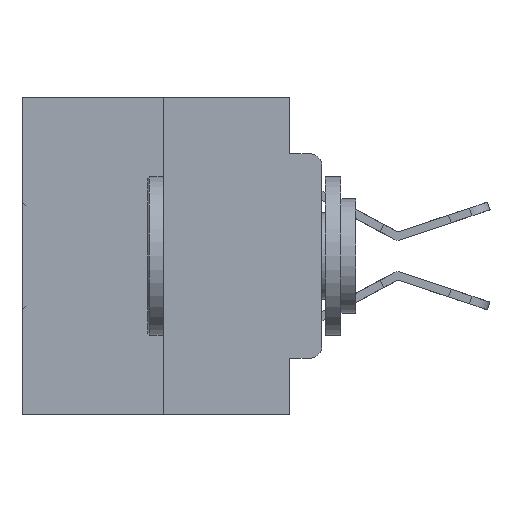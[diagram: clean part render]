
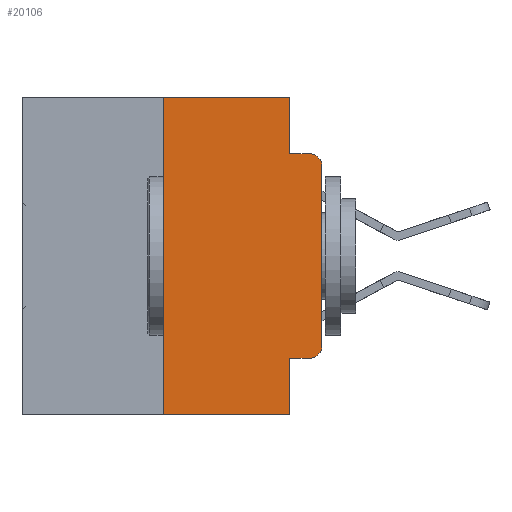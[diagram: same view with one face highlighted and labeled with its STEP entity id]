
A CAD part, left-side view. The second image highlights one B-rep face of the part: STEP entity #20106.
In plain terms, the highlighted planar face has unit normal (-1, 0, 0).
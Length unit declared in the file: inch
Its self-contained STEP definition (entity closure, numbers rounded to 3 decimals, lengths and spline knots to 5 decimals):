
#371 = LINE ( 'NONE', #14412, #5824 ) ;
#836 = LINE ( 'NONE', #15766, #27241 ) ;
#962 = AXIS2_PLACEMENT_3D ( 'NONE', #31679, #16989, #1334 ) ;
#1334 = DIRECTION ( 'NONE',  ( 0., 0., -1. ) ) ;
#1443 = CARTESIAN_POINT ( 'NONE',  ( 0., 0.25, 0. ) ) ;
#1531 = CIRCLE ( 'NONE', #962, 0.02 ) ;
#1955 = ORIENTED_EDGE ( 'NONE', *, *, #29568, .F. ) ;
#3043 = VECTOR ( 'NONE', #22817, 39.37008 ) ;
#3607 = LINE ( 'NONE', #12503, #16623 ) ;
#3695 = DIRECTION ( 'NONE',  ( 0., -1., 0. ) ) ;
#4086 = EDGE_CURVE ( 'NONE', #24337, #12798, #836, .T. ) ;
#4461 = ORIENTED_EDGE ( 'NONE', *, *, #20427, .T. ) ;
#5219 = PLANE ( 'NONE',  #29538 ) ;
#5430 = EDGE_CURVE ( 'NONE', #26293, #6382, #20924, .T. ) ;
#5565 = CARTESIAN_POINT ( 'NONE',  ( 0., 0.02, -0.1085 ) ) ;
#5824 = VECTOR ( 'NONE', #6723, 39.37008 ) ;
#6382 = VERTEX_POINT ( 'NONE', #22737 ) ;
#6723 = DIRECTION ( 'NONE',  ( 0., -1., 0. ) ) ;
#7226 = VECTOR ( 'NONE', #17178, 39.37008 ) ;
#7345 = CIRCLE ( 'NONE', #23878, 0.02 ) ;
#7368 = ORIENTED_EDGE ( 'NONE', *, *, #8764, .F. ) ;
#7575 = CARTESIAN_POINT ( 'NONE',  ( 0., 0.25, 0. ) ) ;
#8210 = DIRECTION ( 'NONE',  ( 0., 0., -1. ) ) ;
#8244 = CARTESIAN_POINT ( 'NONE',  ( 0., 0.051, 0. ) ) ;
#8764 = EDGE_CURVE ( 'NONE', #10915, #15025, #371, .T. ) ;
#9441 = VECTOR ( 'NONE', #12786, 39.37008 ) ;
#9856 = EDGE_CURVE ( 'NONE', #26293, #10915, #29400, .T. ) ;
#9999 = LINE ( 'NONE', #26650, #16008 ) ;
#10063 = LINE ( 'NONE', #20355, #3043 ) ;
#10625 = EDGE_CURVE ( 'NONE', #26866, #32102, #7345, .T. ) ;
#10708 = VERTEX_POINT ( 'NONE', #13634 ) ;
#10915 = VERTEX_POINT ( 'NONE', #1443 ) ;
#11816 = ORIENTED_EDGE ( 'NONE', *, *, #26730, .T. ) ;
#12371 = CARTESIAN_POINT ( 'NONE',  ( 0., 0.473, -0.5 ) ) ;
#12503 = CARTESIAN_POINT ( 'NONE',  ( 0., 0., 0. ) ) ;
#12786 = DIRECTION ( 'NONE',  ( 0., 0., 1. ) ) ;
#12798 = VERTEX_POINT ( 'NONE', #30124 ) ;
#13430 = CARTESIAN_POINT ( 'NONE',  ( 0., 0., -0.3915 ) ) ;
#13448 = ORIENTED_EDGE ( 'NONE', *, *, #17779, .F. ) ;
#13587 = LINE ( 'NONE', #8244, #19589 ) ;
#13634 = CARTESIAN_POINT ( 'NONE',  ( 0., 0.051, -0.0885 ) ) ;
#14412 = CARTESIAN_POINT ( 'NONE',  ( 0., 0.473, 0. ) ) ;
#15025 = VERTEX_POINT ( 'NONE', #18562 ) ;
#15657 = DIRECTION ( 'NONE',  ( 0., 0., -1. ) ) ;
#15766 = CARTESIAN_POINT ( 'NONE',  ( 0., 0.051, -0.4115 ) ) ;
#16008 = VECTOR ( 'NONE', #29107, 39.37008 ) ;
#16623 = VECTOR ( 'NONE', #17682, 39.37008 ) ;
#16989 = DIRECTION ( 'NONE',  ( -1., 0., 0. ) ) ;
#17178 = DIRECTION ( 'NONE',  ( 0., -1., 0. ) ) ;
#17479 = FACE_OUTER_BOUND ( 'NONE', #19697, .T. ) ;
#17682 = DIRECTION ( 'NONE',  ( 0., 0., 1. ) ) ;
#17779 = EDGE_CURVE ( 'NONE', #15025, #10708, #13587, .T. ) ;
#18487 = DIRECTION ( 'NONE',  ( 0., 0., -1. ) ) ;
#18562 = CARTESIAN_POINT ( 'NONE',  ( 0., 0.051, 0. ) ) ;
#19453 = ORIENTED_EDGE ( 'NONE', *, *, #28633, .F. ) ;
#19589 = VECTOR ( 'NONE', #18487, 39.37008 ) ;
#19697 = EDGE_LOOP ( 'NONE', ( #11816, #31633, #19453, #13448, #7368, #21046, #27466, #1955, #29000, #4461 ) ) ;
#20106 = ADVANCED_FACE ( 'NONE', ( #17479 ), #5219, .F. ) ;
#20355 = CARTESIAN_POINT ( 'NONE',  ( 0., 0.051, -0.0885 ) ) ;
#20427 = EDGE_CURVE ( 'NONE', #12798, #22622, #1531, .T. ) ;
#20924 = LINE ( 'NONE', #12371, #7226 ) ;
#20938 = CARTESIAN_POINT ( 'NONE',  ( 0., 0.25, -0.5 ) ) ;
#21046 = ORIENTED_EDGE ( 'NONE', *, *, #9856, .F. ) ;
#22622 = VERTEX_POINT ( 'NONE', #13430 ) ;
#22737 = CARTESIAN_POINT ( 'NONE',  ( 0., 0.051, -0.5 ) ) ;
#22817 = DIRECTION ( 'NONE',  ( 0., -1., 0. ) ) ;
#23448 = DIRECTION ( 'NONE',  ( -1., 0., 0. ) ) ;
#23878 = AXIS2_PLACEMENT_3D ( 'NONE', #5565, #23448, #8210 ) ;
#24337 = VERTEX_POINT ( 'NONE', #27495 ) ;
#25555 = CARTESIAN_POINT ( 'NONE',  ( 0., 0.473, 0. ) ) ;
#26293 = VERTEX_POINT ( 'NONE', #20938 ) ;
#26650 = CARTESIAN_POINT ( 'NONE',  ( 0., 0.051, 0. ) ) ;
#26730 = EDGE_CURVE ( 'NONE', #22622, #26866, #3607, .T. ) ;
#26866 = VERTEX_POINT ( 'NONE', #30327 ) ;
#27241 = VECTOR ( 'NONE', #3695, 39.37008 ) ;
#27466 = ORIENTED_EDGE ( 'NONE', *, *, #5430, .T. ) ;
#27495 = CARTESIAN_POINT ( 'NONE',  ( 0., 0.051, -0.4115 ) ) ;
#28633 = EDGE_CURVE ( 'NONE', #10708, #32102, #10063, .T. ) ;
#29000 = ORIENTED_EDGE ( 'NONE', *, *, #4086, .T. ) ;
#29107 = DIRECTION ( 'NONE',  ( 0., 0., -1. ) ) ;
#29400 = LINE ( 'NONE', #7575, #9441 ) ;
#29538 = AXIS2_PLACEMENT_3D ( 'NONE', #25555, #30437, #15657 ) ;
#29568 = EDGE_CURVE ( 'NONE', #24337, #6382, #9999, .T. ) ;
#30124 = CARTESIAN_POINT ( 'NONE',  ( 0., 0.02, -0.4115 ) ) ;
#30327 = CARTESIAN_POINT ( 'NONE',  ( 0., 0., -0.1085 ) ) ;
#30437 = DIRECTION ( 'NONE',  ( 1., 0., 0. ) ) ;
#31633 = ORIENTED_EDGE ( 'NONE', *, *, #10625, .T. ) ;
#31679 = CARTESIAN_POINT ( 'NONE',  ( 0., 0.02, -0.3915 ) ) ;
#32102 = VERTEX_POINT ( 'NONE', #32621 ) ;
#32621 = CARTESIAN_POINT ( 'NONE',  ( 0., 0.02, -0.0885 ) ) ;
